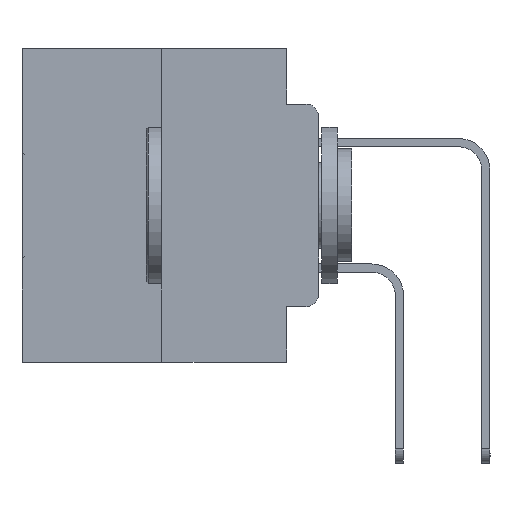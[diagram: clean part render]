
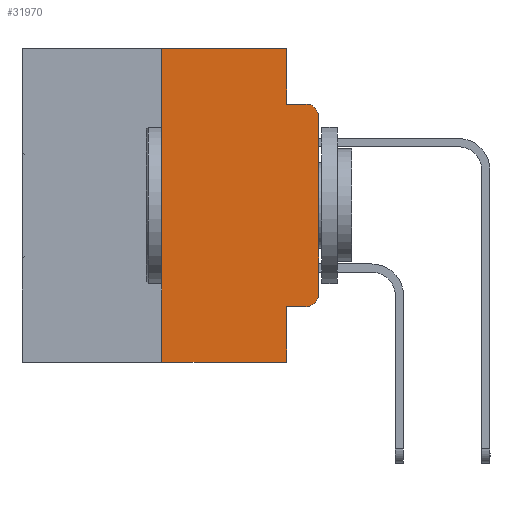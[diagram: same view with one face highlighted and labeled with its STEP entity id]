
A CAD part, left-side view. The second image highlights one B-rep face of the part: STEP entity #31970.
In plain terms, the highlighted planar face has unit normal (-1, 0, 0).
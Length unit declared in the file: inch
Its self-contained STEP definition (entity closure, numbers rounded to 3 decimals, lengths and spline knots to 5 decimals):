
#223 = ORIENTED_EDGE ( 'NONE', *, *, #16401, .F. ) ;
#386 = CARTESIAN_POINT ( 'NONE',  ( 0., 0.02, -0.3915 ) ) ;
#627 = VECTOR ( 'NONE', #31844, 39.37008 ) ;
#1206 = VERTEX_POINT ( 'NONE', #17570 ) ;
#1459 = CARTESIAN_POINT ( 'NONE',  ( 0., 0.25, 0. ) ) ;
#2002 = DIRECTION ( 'NONE',  ( 0., -1., 0. ) ) ;
#2716 = ORIENTED_EDGE ( 'NONE', *, *, #10174, .F. ) ;
#2724 = ORIENTED_EDGE ( 'NONE', *, *, #31523, .F. ) ;
#2909 = VERTEX_POINT ( 'NONE', #26853 ) ;
#3662 = VERTEX_POINT ( 'NONE', #4790 ) ;
#4077 = LINE ( 'NONE', #1459, #17032 ) ;
#4730 = VECTOR ( 'NONE', #23946, 39.37008 ) ;
#4790 = CARTESIAN_POINT ( 'NONE',  ( 0., 0.25, 0. ) ) ;
#5229 = VECTOR ( 'NONE', #2002, 39.37008 ) ;
#6522 = CARTESIAN_POINT ( 'NONE',  ( 0., 0.051, -0.0885 ) ) ;
#6894 = EDGE_LOOP ( 'NONE', ( #11498, #15228, #2724, #13451, #223, #2716, #28288, #16035, #15272, #14143 ) ) ;
#7063 = LINE ( 'NONE', #8908, #627 ) ;
#7072 = CARTESIAN_POINT ( 'NONE',  ( 0., 0.051, -0.4115 ) ) ;
#7153 = CARTESIAN_POINT ( 'NONE',  ( 0., 0.25, -0.5 ) ) ;
#7420 = DIRECTION ( 'NONE',  ( 0., 0., -1. ) ) ;
#7470 = CARTESIAN_POINT ( 'NONE',  ( 0., 0.02, -0.0885 ) ) ;
#7980 = VERTEX_POINT ( 'NONE', #9359 ) ;
#8302 = DIRECTION ( 'NONE',  ( -1., 0., 0. ) ) ;
#8908 = CARTESIAN_POINT ( 'NONE',  ( 0., 0.473, 0. ) ) ;
#9359 = CARTESIAN_POINT ( 'NONE',  ( 0., 0.02, -0.4115 ) ) ;
#9481 = LINE ( 'NONE', #32141, #13977 ) ;
#10174 = EDGE_CURVE ( 'NONE', #24274, #3662, #4077, .T. ) ;
#11130 = DIRECTION ( 'NONE',  ( 0., -1., 0. ) ) ;
#11418 = DIRECTION ( 'NONE',  ( 0., 0., 1. ) ) ;
#11498 = ORIENTED_EDGE ( 'NONE', *, *, #16978, .T. ) ;
#12401 = DIRECTION ( 'NONE',  ( 0., 0., -1. ) ) ;
#12752 = VERTEX_POINT ( 'NONE', #7470 ) ;
#13267 = CARTESIAN_POINT ( 'NONE',  ( 0., 0., -0.3915 ) ) ;
#13451 = ORIENTED_EDGE ( 'NONE', *, *, #16447, .F. ) ;
#13501 = DIRECTION ( 'NONE',  ( 0., 0., -1. ) ) ;
#13977 = VECTOR ( 'NONE', #12401, 39.37008 ) ;
#14143 = ORIENTED_EDGE ( 'NONE', *, *, #22532, .T. ) ;
#14598 = DIRECTION ( 'NONE',  ( -1., 0., 0. ) ) ;
#14703 = EDGE_CURVE ( 'NONE', #23571, #7980, #24012, .T. ) ;
#14805 = CIRCLE ( 'NONE', #21481, 0.02 ) ;
#14998 = CARTESIAN_POINT ( 'NONE',  ( 0., 0., 0. ) ) ;
#15228 = ORIENTED_EDGE ( 'NONE', *, *, #21886, .T. ) ;
#15272 = ORIENTED_EDGE ( 'NONE', *, *, #14703, .T. ) ;
#15946 = DIRECTION ( 'NONE',  ( 0., 0., -1. ) ) ;
#16035 = ORIENTED_EDGE ( 'NONE', *, *, #29784, .F. ) ;
#16180 = AXIS2_PLACEMENT_3D ( 'NONE', #20840, #30799, #13501 ) ;
#16401 = EDGE_CURVE ( 'NONE', #3662, #2909, #7063, .T. ) ;
#16447 = EDGE_CURVE ( 'NONE', #2909, #29977, #27285, .T. ) ;
#16978 = EDGE_CURVE ( 'NONE', #27856, #1206, #19734, .T. ) ;
#17032 = VECTOR ( 'NONE', #11418, 39.37008 ) ;
#17570 = CARTESIAN_POINT ( 'NONE',  ( 0., 0., -0.1085 ) ) ;
#17640 = CARTESIAN_POINT ( 'NONE',  ( 0., 0.051, 0. ) ) ;
#18226 = PLANE ( 'NONE',  #16180 ) ;
#18362 = CIRCLE ( 'NONE', #30384, 0.02 ) ;
#18463 = LINE ( 'NONE', #18942, #25408 ) ;
#18942 = CARTESIAN_POINT ( 'NONE',  ( 0., 0.473, -0.5 ) ) ;
#19253 = VERTEX_POINT ( 'NONE', #23376 ) ;
#19734 = LINE ( 'NONE', #14998, #23562 ) ;
#20265 = DIRECTION ( 'NONE',  ( 0., 0., -1. ) ) ;
#20840 = CARTESIAN_POINT ( 'NONE',  ( 0., 0.473, 0. ) ) ;
#21481 = AXIS2_PLACEMENT_3D ( 'NONE', #26061, #8302, #15946 ) ;
#21886 = EDGE_CURVE ( 'NONE', #1206, #12752, #14805, .T. ) ;
#22532 = EDGE_CURVE ( 'NONE', #7980, #27856, #18362, .T. ) ;
#23376 = CARTESIAN_POINT ( 'NONE',  ( 0., 0.051, -0.5 ) ) ;
#23562 = VECTOR ( 'NONE', #29709, 39.37008 ) ;
#23571 = VERTEX_POINT ( 'NONE', #28179 ) ;
#23946 = DIRECTION ( 'NONE',  ( 0., -1., 0. ) ) ;
#24012 = LINE ( 'NONE', #7072, #5229 ) ;
#24274 = VERTEX_POINT ( 'NONE', #7153 ) ;
#25408 = VECTOR ( 'NONE', #11130, 39.37008 ) ;
#25597 = CARTESIAN_POINT ( 'NONE',  ( 0., 0.051, -0.0885 ) ) ;
#26061 = CARTESIAN_POINT ( 'NONE',  ( 0., 0.02, -0.1085 ) ) ;
#26256 = LINE ( 'NONE', #6522, #4730 ) ;
#26853 = CARTESIAN_POINT ( 'NONE',  ( 0., 0.051, 0. ) ) ;
#27285 = LINE ( 'NONE', #17640, #27749 ) ;
#27749 = VECTOR ( 'NONE', #20265, 39.37008 ) ;
#27856 = VERTEX_POINT ( 'NONE', #13267 ) ;
#28179 = CARTESIAN_POINT ( 'NONE',  ( 0., 0.051, -0.4115 ) ) ;
#28288 = ORIENTED_EDGE ( 'NONE', *, *, #29701, .T. ) ;
#29701 = EDGE_CURVE ( 'NONE', #24274, #19253, #18463, .T. ) ;
#29709 = DIRECTION ( 'NONE',  ( 0., 0., 1. ) ) ;
#29784 = EDGE_CURVE ( 'NONE', #23571, #19253, #9481, .T. ) ;
#29977 = VERTEX_POINT ( 'NONE', #25597 ) ;
#30384 = AXIS2_PLACEMENT_3D ( 'NONE', #386, #14598, #7420 ) ;
#30799 = DIRECTION ( 'NONE',  ( 1., 0., 0. ) ) ;
#31440 = FACE_OUTER_BOUND ( 'NONE', #6894, .T. ) ;
#31523 = EDGE_CURVE ( 'NONE', #29977, #12752, #26256, .T. ) ;
#31844 = DIRECTION ( 'NONE',  ( 0., -1., 0. ) ) ;
#31970 = ADVANCED_FACE ( 'NONE', ( #31440 ), #18226, .F. ) ;
#32141 = CARTESIAN_POINT ( 'NONE',  ( 0., 0.051, 0. ) ) ;
